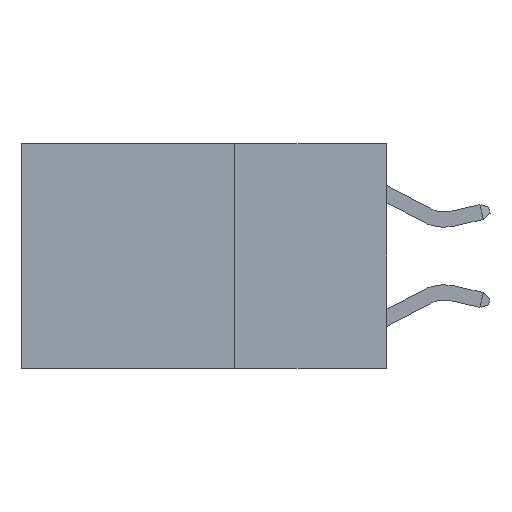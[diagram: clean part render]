
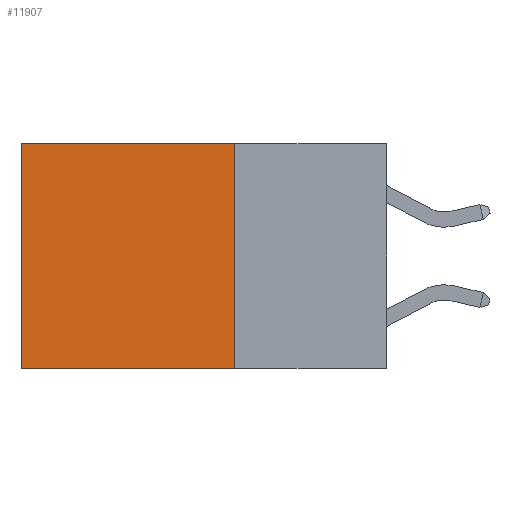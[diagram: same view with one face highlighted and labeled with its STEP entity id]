
A CAD part, left-side view. The second image highlights one B-rep face of the part: STEP entity #11907.
In plain terms, the highlighted planar face has unit normal (-1, 0, 0).
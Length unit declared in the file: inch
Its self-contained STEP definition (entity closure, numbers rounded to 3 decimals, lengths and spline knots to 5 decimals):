
#1248 = DIRECTION ( 'NONE',  ( 0., 1., 0. ) ) ;
#1286 = AXIS2_PLACEMENT_3D ( 'NONE', #3250, #11602, #13212 ) ;
#1397 = VERTEX_POINT ( 'NONE', #3598 ) ;
#1448 = CARTESIAN_POINT ( 'NONE',  ( 0.2625, 0.6, 0. ) ) ;
#1759 = ORIENTED_EDGE ( 'NONE', *, *, #10561, .T. ) ;
#2313 = CARTESIAN_POINT ( 'NONE',  ( 0.2625, 0.6, 0. ) ) ;
#2694 = EDGE_CURVE ( 'NONE', #8045, #1397, #11134, .T. ) ;
#2960 = DIRECTION ( 'NONE',  ( 0., 0., -1. ) ) ;
#3250 = CARTESIAN_POINT ( 'NONE',  ( 0.2625, 0.25, 0. ) ) ;
#3598 = CARTESIAN_POINT ( 'NONE',  ( 0.2625, 0.25, -0.37 ) ) ;
#4605 = EDGE_CURVE ( 'NONE', #1397, #9960, #12914, .T. ) ;
#5937 = ORIENTED_EDGE ( 'NONE', *, *, #2694, .F. ) ;
#7314 = PLANE ( 'NONE',  #1286 ) ;
#7509 = VECTOR ( 'NONE', #1248, 39.37008 ) ;
#8045 = VERTEX_POINT ( 'NONE', #18567 ) ;
#8106 = CARTESIAN_POINT ( 'NONE',  ( 0.2625, 0.25, -0.37 ) ) ;
#8288 = DIRECTION ( 'NONE',  ( 0., 1., 0. ) ) ;
#8608 = VECTOR ( 'NONE', #8288, 39.37008 ) ;
#8938 = EDGE_LOOP ( 'NONE', ( #1759, #17082, #5937, #17929 ) ) ;
#9032 = LINE ( 'NONE', #1448, #9836 ) ;
#9836 = VECTOR ( 'NONE', #2960, 39.37008 ) ;
#9960 = VERTEX_POINT ( 'NONE', #10655 ) ;
#10107 = VERTEX_POINT ( 'NONE', #2313 ) ;
#10561 = EDGE_CURVE ( 'NONE', #10107, #9960, #9032, .T. ) ;
#10655 = CARTESIAN_POINT ( 'NONE',  ( 0.2625, 0.6, -0.37 ) ) ;
#11134 = LINE ( 'NONE', #18282, #16331 ) ;
#11137 = LINE ( 'NONE', #16954, #8608 ) ;
#11602 = DIRECTION ( 'NONE',  ( 1., 0., 0. ) ) ;
#11907 = ADVANCED_FACE ( 'NONE', ( #17502 ), #7314, .F. ) ;
#12193 = DIRECTION ( 'NONE',  ( 0., 0., -1. ) ) ;
#12914 = LINE ( 'NONE', #8106, #7509 ) ;
#13212 = DIRECTION ( 'NONE',  ( 0., 0., -1. ) ) ;
#15951 = EDGE_CURVE ( 'NONE', #8045, #10107, #11137, .T. ) ;
#16331 = VECTOR ( 'NONE', #12193, 39.37008 ) ;
#16954 = CARTESIAN_POINT ( 'NONE',  ( 0.2625, 0.25, 0. ) ) ;
#17082 = ORIENTED_EDGE ( 'NONE', *, *, #4605, .F. ) ;
#17502 = FACE_OUTER_BOUND ( 'NONE', #8938, .T. ) ;
#17929 = ORIENTED_EDGE ( 'NONE', *, *, #15951, .T. ) ;
#18282 = CARTESIAN_POINT ( 'NONE',  ( 0.2625, 0.25, 0. ) ) ;
#18567 = CARTESIAN_POINT ( 'NONE',  ( 0.2625, 0.25, 0. ) ) ;
